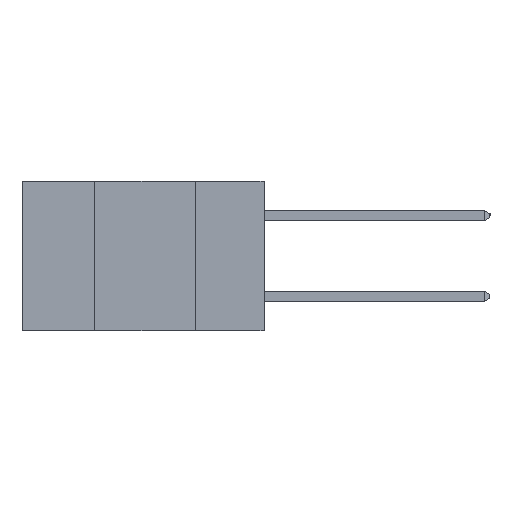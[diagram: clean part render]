
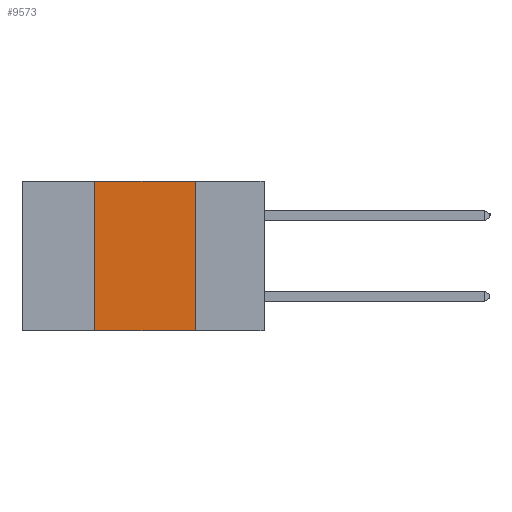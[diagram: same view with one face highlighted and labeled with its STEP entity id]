
A CAD part, left-side view. The second image highlights one B-rep face of the part: STEP entity #9573.
In plain terms, the highlighted planar face has unit normal (-1, 0, 0).
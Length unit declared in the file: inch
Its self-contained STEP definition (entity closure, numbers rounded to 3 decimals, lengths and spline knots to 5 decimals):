
#260 = CARTESIAN_POINT ( 'NONE',  ( 0., 0.6, 0. ) ) ;
#898 = ORIENTED_EDGE ( 'NONE', *, *, #10521, .F. ) ;
#1499 = VERTEX_POINT ( 'NONE', #3630 ) ;
#1547 = DIRECTION ( 'NONE',  ( 1., 0., 0. ) ) ;
#2134 = CARTESIAN_POINT ( 'NONE',  ( 0., 0.6, -0.37 ) ) ;
#2795 = VERTEX_POINT ( 'NONE', #6648 ) ;
#3460 = DIRECTION ( 'NONE',  ( 0., 0., -1. ) ) ;
#3630 = CARTESIAN_POINT ( 'NONE',  ( 0., 0.42, 0. ) ) ;
#3781 = EDGE_CURVE ( 'NONE', #1499, #10694, #5744, .T. ) ;
#3794 = VECTOR ( 'NONE', #3851, 39.37008 ) ;
#3851 = DIRECTION ( 'NONE',  ( 0., -1., 0. ) ) ;
#3958 = VECTOR ( 'NONE', #10407, 39.37008 ) ;
#4082 = LINE ( 'NONE', #5103, #12582 ) ;
#4642 = ORIENTED_EDGE ( 'NONE', *, *, #3781, .F. ) ;
#4790 = CARTESIAN_POINT ( 'NONE',  ( 0., 0.6, 0. ) ) ;
#4988 = VERTEX_POINT ( 'NONE', #11630 ) ;
#5103 = CARTESIAN_POINT ( 'NONE',  ( 0., 0.17, -0.37 ) ) ;
#5203 = CARTESIAN_POINT ( 'NONE',  ( 0., 0.17, 0. ) ) ;
#5744 = LINE ( 'NONE', #4790, #3794 ) ;
#6090 = CARTESIAN_POINT ( 'NONE',  ( 0., 0.42, -0.37 ) ) ;
#6297 = EDGE_LOOP ( 'NONE', ( #11518, #4642, #898, #6904 ) ) ;
#6379 = LINE ( 'NONE', #2134, #3958 ) ;
#6648 = CARTESIAN_POINT ( 'NONE',  ( 0., 0.42, -0.37 ) ) ;
#6838 = DIRECTION ( 'NONE',  ( 0., 0., 1. ) ) ;
#6904 = ORIENTED_EDGE ( 'NONE', *, *, #9894, .T. ) ;
#7417 = FACE_OUTER_BOUND ( 'NONE', #6297, .T. ) ;
#8031 = LINE ( 'NONE', #6090, #11678 ) ;
#8217 = AXIS2_PLACEMENT_3D ( 'NONE', #260, #1547, #3460 ) ;
#8422 = PLANE ( 'NONE',  #8217 ) ;
#9392 = DIRECTION ( 'NONE',  ( 0., 0., -1. ) ) ;
#9573 = ADVANCED_FACE ( 'NONE', ( #7417 ), #8422, .F. ) ;
#9894 = EDGE_CURVE ( 'NONE', #2795, #4988, #6379, .T. ) ;
#10407 = DIRECTION ( 'NONE',  ( 0., -1., 0. ) ) ;
#10521 = EDGE_CURVE ( 'NONE', #2795, #1499, #8031, .T. ) ;
#10694 = VERTEX_POINT ( 'NONE', #5203 ) ;
#11518 = ORIENTED_EDGE ( 'NONE', *, *, #13284, .F. ) ;
#11630 = CARTESIAN_POINT ( 'NONE',  ( 0., 0.17, -0.37 ) ) ;
#11678 = VECTOR ( 'NONE', #6838, 39.37008 ) ;
#12582 = VECTOR ( 'NONE', #9392, 39.37008 ) ;
#13284 = EDGE_CURVE ( 'NONE', #10694, #4988, #4082, .T. ) ;
